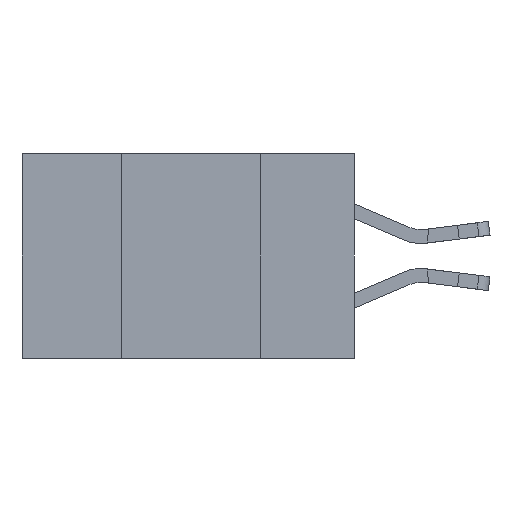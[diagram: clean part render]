
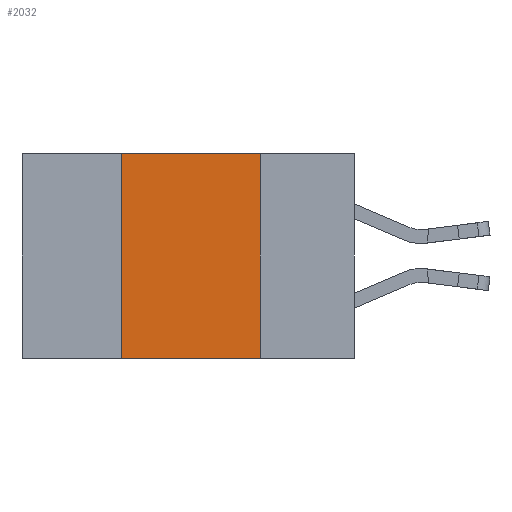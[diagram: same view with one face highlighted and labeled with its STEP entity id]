
A CAD part, left-side view. The second image highlights one B-rep face of the part: STEP entity #2032.
In plain terms, the highlighted planar face has unit normal (-1, 0, 0).
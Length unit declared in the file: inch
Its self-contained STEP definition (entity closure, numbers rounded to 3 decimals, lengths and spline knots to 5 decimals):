
#1282 = DIRECTION ( 'NONE',  ( 1., 0., 0. ) ) ;
#1349 = DIRECTION ( 'NONE',  ( 0., 0., -1. ) ) ;
#1572 = CARTESIAN_POINT ( 'NONE',  ( 0., 0.6, 0. ) ) ;
#1638 = CARTESIAN_POINT ( 'NONE',  ( 0., 0.6, -0.37 ) ) ;
#1687 = VERTEX_POINT ( 'NONE', #9790 ) ;
#1774 = LINE ( 'NONE', #10090, #6383 ) ;
#1777 = CARTESIAN_POINT ( 'NONE',  ( 0., 0.17, -0.37 ) ) ;
#2032 = ADVANCED_FACE ( 'NONE', ( #5481 ), #10608, .F. ) ;
#2158 = VECTOR ( 'NONE', #10721, 39.37008 ) ;
#3130 = DIRECTION ( 'NONE',  ( 0., -1., 0. ) ) ;
#3698 = EDGE_CURVE ( 'NONE', #13302, #14961, #1774, .T. ) ;
#5274 = EDGE_LOOP ( 'NONE', ( #18346, #13334, #10140, #7617 ) ) ;
#5310 = DIRECTION ( 'NONE',  ( 0., 0., 1. ) ) ;
#5481 = FACE_OUTER_BOUND ( 'NONE', #5274, .T. ) ;
#6383 = VECTOR ( 'NONE', #5310, 39.37008 ) ;
#7258 = LINE ( 'NONE', #13851, #2158 ) ;
#7313 = CARTESIAN_POINT ( 'NONE',  ( 0., 0.42, -0.37 ) ) ;
#7379 = CARTESIAN_POINT ( 'NONE',  ( 0., 0.6, 0. ) ) ;
#7617 = ORIENTED_EDGE ( 'NONE', *, *, #10719, .T. ) ;
#8953 = VECTOR ( 'NONE', #13887, 39.37008 ) ;
#9790 = CARTESIAN_POINT ( 'NONE',  ( 0., 0.17, 0. ) ) ;
#10090 = CARTESIAN_POINT ( 'NONE',  ( 0., 0.42, 0. ) ) ;
#10140 = ORIENTED_EDGE ( 'NONE', *, *, #3698, .F. ) ;
#10608 = PLANE ( 'NONE',  #12673 ) ;
#10719 = EDGE_CURVE ( 'NONE', #13302, #16185, #13076, .T. ) ;
#10721 = DIRECTION ( 'NONE',  ( 0., 0., -1. ) ) ;
#11904 = LINE ( 'NONE', #1572, #14547 ) ;
#12673 = AXIS2_PLACEMENT_3D ( 'NONE', #7379, #1282, #1349 ) ;
#13076 = LINE ( 'NONE', #1638, #8953 ) ;
#13302 = VERTEX_POINT ( 'NONE', #7313 ) ;
#13334 = ORIENTED_EDGE ( 'NONE', *, *, #14186, .F. ) ;
#13851 = CARTESIAN_POINT ( 'NONE',  ( 0., 0.17, 0. ) ) ;
#13887 = DIRECTION ( 'NONE',  ( 0., -1., 0. ) ) ;
#14186 = EDGE_CURVE ( 'NONE', #14961, #1687, #11904, .T. ) ;
#14547 = VECTOR ( 'NONE', #3130, 39.37008 ) ;
#14961 = VERTEX_POINT ( 'NONE', #18645 ) ;
#15319 = EDGE_CURVE ( 'NONE', #1687, #16185, #7258, .T. ) ;
#16185 = VERTEX_POINT ( 'NONE', #1777 ) ;
#18346 = ORIENTED_EDGE ( 'NONE', *, *, #15319, .F. ) ;
#18645 = CARTESIAN_POINT ( 'NONE',  ( 0., 0.42, 0. ) ) ;
